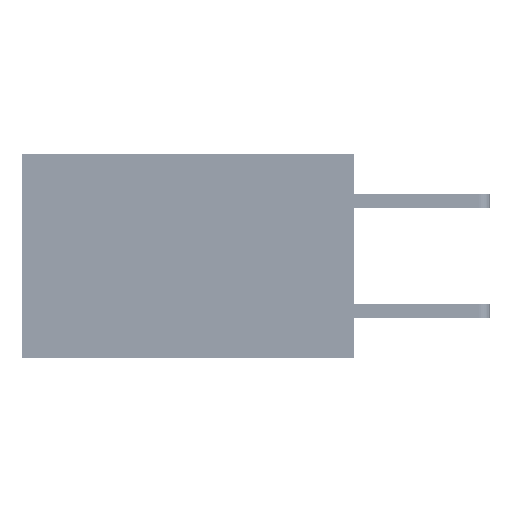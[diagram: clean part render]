
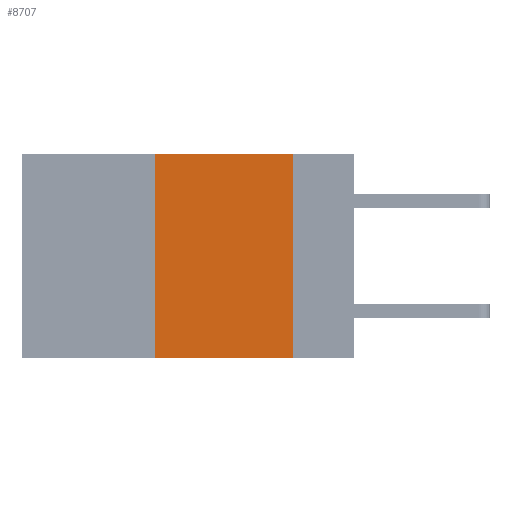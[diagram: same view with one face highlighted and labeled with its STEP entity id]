
A CAD part, left-side view. The second image highlights one B-rep face of the part: STEP entity #8707.
In plain terms, the highlighted planar face has unit normal (-1, 0, 0).
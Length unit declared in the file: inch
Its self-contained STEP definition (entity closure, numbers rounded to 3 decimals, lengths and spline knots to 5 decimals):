
#473 = VERTEX_POINT ( 'NONE', #27837 ) ;
#2118 = PLANE ( 'NONE',  #37618 ) ;
#2426 = DIRECTION ( 'NONE',  ( 0., -1., 0. ) ) ;
#3001 = CARTESIAN_POINT ( 'NONE',  ( 0., 0.6, 0. ) ) ;
#3251 = VECTOR ( 'NONE', #34568, 39.37008 ) ;
#3546 = VERTEX_POINT ( 'NONE', #10258 ) ;
#7111 = CARTESIAN_POINT ( 'NONE',  ( 0., 0.36, 0. ) ) ;
#8707 = ADVANCED_FACE ( 'NONE', ( #43248 ), #2118, .F. ) ;
#10258 = CARTESIAN_POINT ( 'NONE',  ( 0., 0.11, -0.37 ) ) ;
#13051 = CARTESIAN_POINT ( 'NONE',  ( 0., 0.11, 0. ) ) ;
#13518 = CARTESIAN_POINT ( 'NONE',  ( 0., 0.6, -0.37 ) ) ;
#16891 = EDGE_CURVE ( 'NONE', #22319, #3546, #35052, .T. ) ;
#19445 = ORIENTED_EDGE ( 'NONE', *, *, #46687, .T. ) ;
#20669 = ORIENTED_EDGE ( 'NONE', *, *, #23169, .F. ) ;
#21664 = LINE ( 'NONE', #7111, #47956 ) ;
#22319 = VERTEX_POINT ( 'NONE', #13051 ) ;
#22636 = VECTOR ( 'NONE', #2426, 39.37008 ) ;
#23169 = EDGE_CURVE ( 'NONE', #473, #22319, #40446, .T. ) ;
#24051 = DIRECTION ( 'NONE',  ( 1., 0., 0. ) ) ;
#24861 = EDGE_LOOP ( 'NONE', ( #30063, #20669, #39913, #19445 ) ) ;
#27837 = CARTESIAN_POINT ( 'NONE',  ( 0., 0.36, 0. ) ) ;
#28044 = LINE ( 'NONE', #13518, #22636 ) ;
#30063 = ORIENTED_EDGE ( 'NONE', *, *, #16891, .F. ) ;
#34568 = DIRECTION ( 'NONE',  ( 0., 0., -1. ) ) ;
#35052 = LINE ( 'NONE', #35291, #3251 ) ;
#35291 = CARTESIAN_POINT ( 'NONE',  ( 0., 0.11, 0. ) ) ;
#36414 = VERTEX_POINT ( 'NONE', #41165 ) ;
#36506 = DIRECTION ( 'NONE',  ( 0., -1., 0. ) ) ;
#37618 = AXIS2_PLACEMENT_3D ( 'NONE', #39557, #24051, #39054 ) ;
#39054 = DIRECTION ( 'NONE',  ( 0., 0., -1. ) ) ;
#39557 = CARTESIAN_POINT ( 'NONE',  ( 0., 0.6, 0. ) ) ;
#39913 = ORIENTED_EDGE ( 'NONE', *, *, #48603, .F. ) ;
#40446 = LINE ( 'NONE', #3001, #42857 ) ;
#41165 = CARTESIAN_POINT ( 'NONE',  ( 0., 0.36, -0.37 ) ) ;
#42857 = VECTOR ( 'NONE', #36506, 39.37008 ) ;
#43248 = FACE_OUTER_BOUND ( 'NONE', #24861, .T. ) ;
#46687 = EDGE_CURVE ( 'NONE', #36414, #3546, #28044, .T. ) ;
#47956 = VECTOR ( 'NONE', #48486, 39.37008 ) ;
#48486 = DIRECTION ( 'NONE',  ( 0., 0., 1. ) ) ;
#48603 = EDGE_CURVE ( 'NONE', #36414, #473, #21664, .T. ) ;
